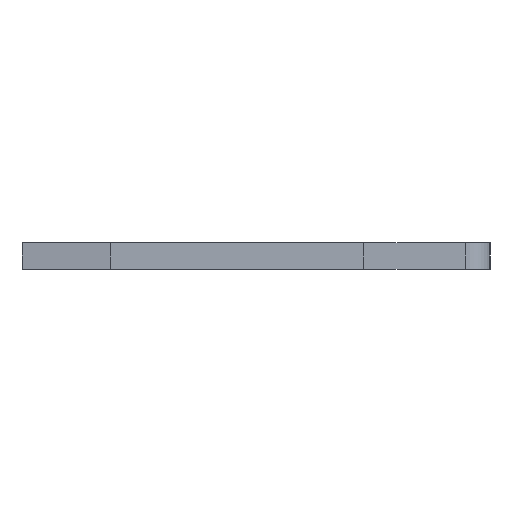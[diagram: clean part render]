
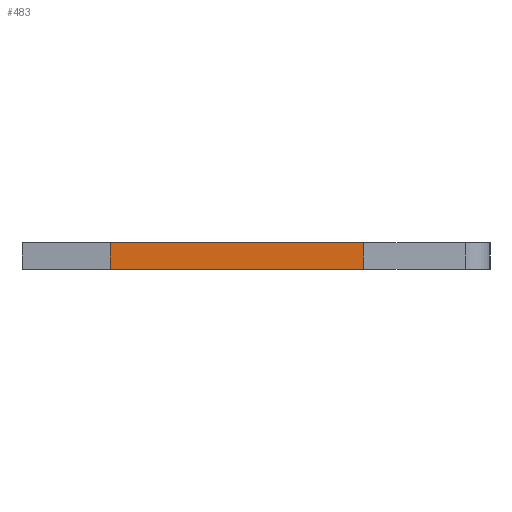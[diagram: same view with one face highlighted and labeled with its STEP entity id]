
A CAD part, left-side view. The second image highlights one B-rep face of the part: STEP entity #483.
In plain terms, the highlighted face is planar.
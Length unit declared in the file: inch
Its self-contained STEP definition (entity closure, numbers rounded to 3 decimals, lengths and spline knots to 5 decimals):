
#25 = AXIS2_PLACEMENT_3D ( 'NONE', #246, #937, #1028 ) ;
#27 = EDGE_CURVE ( 'NONE', #263, #568, #464, .T. ) ;
#88 = VECTOR ( 'NONE', #982, 39.37008 ) ;
#108 = LINE ( 'NONE', #925, #923 ) ;
#167 = LINE ( 'NONE', #829, #892 ) ;
#215 = CARTESIAN_POINT ( 'NONE',  ( 0.013, 0.146, -0.0575 ) ) ;
#246 = CARTESIAN_POINT ( 'NONE',  ( 0.013, 0.146, -0.0575 ) ) ;
#250 = PLANE ( 'NONE',  #25 ) ;
#263 = VERTEX_POINT ( 'NONE', #478 ) ;
#301 = DIRECTION ( 'NONE',  ( 0., 1., 0. ) ) ;
#312 = ORIENTED_EDGE ( 'NONE', *, *, #27, .T. ) ;
#347 = EDGE_CURVE ( 'NONE', #618, #1022, #167, .T. ) ;
#366 = EDGE_LOOP ( 'NONE', ( #837, #1151, #940, #312 ) ) ;
#400 = DIRECTION ( 'NONE',  ( 0., 1., 0. ) ) ;
#457 = VECTOR ( 'NONE', #301, 39.37008 ) ;
#464 = LINE ( 'NONE', #1164, #88 ) ;
#478 = CARTESIAN_POINT ( 'NONE',  ( 0.013, -0.099, -0.0575 ) ) ;
#483 = ADVANCED_FACE ( 'NONE', ( #709 ), #250, .F. ) ;
#568 = VERTEX_POINT ( 'NONE', #1026 ) ;
#572 = DIRECTION ( 'NONE',  ( -1., 0., 0. ) ) ;
#618 = VERTEX_POINT ( 'NONE', #685 ) ;
#685 = CARTESIAN_POINT ( 'NONE',  ( 0.013, 0.146, -0.0575 ) ) ;
#709 = FACE_OUTER_BOUND ( 'NONE', #366, .T. ) ;
#794 = LINE ( 'NONE', #215, #457 ) ;
#829 = CARTESIAN_POINT ( 'NONE',  ( 0.013, 0.146, -0.0575 ) ) ;
#837 = ORIENTED_EDGE ( 'NONE', *, *, #1126, .T. ) ;
#892 = VECTOR ( 'NONE', #572, 39.37008 ) ;
#923 = VECTOR ( 'NONE', #400, 39.37008 ) ;
#925 = CARTESIAN_POINT ( 'NONE',  ( -0.013, 0.146, -0.0575 ) ) ;
#937 = DIRECTION ( 'NONE',  ( 0., 0., 1. ) ) ;
#940 = ORIENTED_EDGE ( 'NONE', *, *, #1051, .F. ) ;
#982 = DIRECTION ( 'NONE',  ( -1., 0., 0. ) ) ;
#1006 = CARTESIAN_POINT ( 'NONE',  ( -0.013, 0.146, -0.0575 ) ) ;
#1022 = VERTEX_POINT ( 'NONE', #1006 ) ;
#1026 = CARTESIAN_POINT ( 'NONE',  ( -0.013, -0.099, -0.0575 ) ) ;
#1028 = DIRECTION ( 'NONE',  ( 1., 0., 0. ) ) ;
#1051 = EDGE_CURVE ( 'NONE', #263, #618, #794, .T. ) ;
#1126 = EDGE_CURVE ( 'NONE', #568, #1022, #108, .T. ) ;
#1151 = ORIENTED_EDGE ( 'NONE', *, *, #347, .F. ) ;
#1164 = CARTESIAN_POINT ( 'NONE',  ( 0.013, -0.099, -0.0575 ) ) ;
